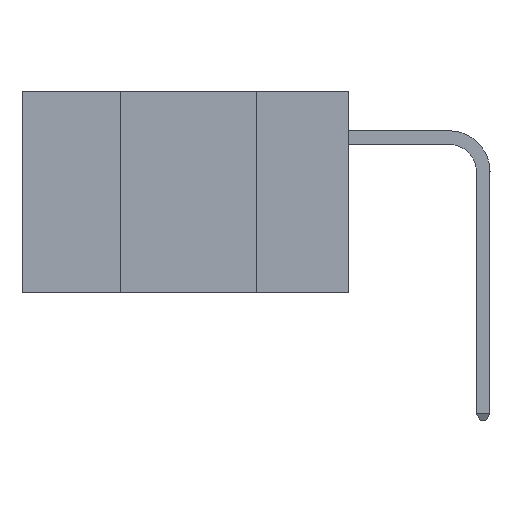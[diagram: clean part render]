
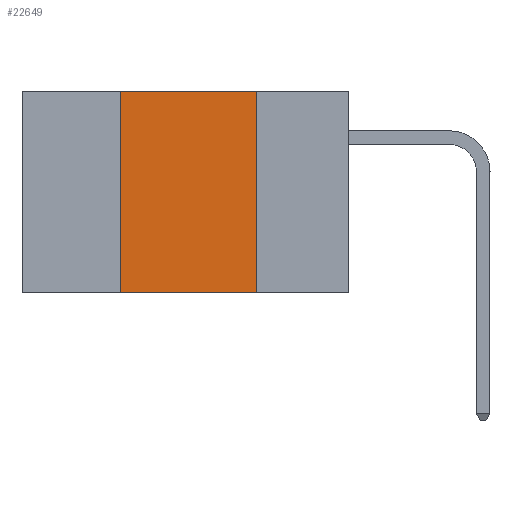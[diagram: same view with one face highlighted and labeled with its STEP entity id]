
A CAD part, left-side view. The second image highlights one B-rep face of the part: STEP entity #22649.
In plain terms, the highlighted planar face has unit normal (-1, 0, 0).
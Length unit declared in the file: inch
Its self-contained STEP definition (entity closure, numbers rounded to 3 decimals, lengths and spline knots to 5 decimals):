
#1308 = EDGE_CURVE ( 'NONE', #11373, #8260, #6706, .T. ) ;
#1594 = DIRECTION ( 'NONE',  ( 0., 0., -1. ) ) ;
#3029 = CARTESIAN_POINT ( 'NONE',  ( 0., 0.42, 0. ) ) ;
#3291 = VECTOR ( 'NONE', #25698, 39.37008 ) ;
#3367 = FACE_OUTER_BOUND ( 'NONE', #34215, .T. ) ;
#3496 = VERTEX_POINT ( 'NONE', #15528 ) ;
#5189 = ORIENTED_EDGE ( 'NONE', *, *, #33796, .F. ) ;
#6593 = DIRECTION ( 'NONE',  ( 0., -1., 0. ) ) ;
#6706 = LINE ( 'NONE', #19530, #32050 ) ;
#7103 = ORIENTED_EDGE ( 'NONE', *, *, #1308, .F. ) ;
#8260 = VERTEX_POINT ( 'NONE', #3029 ) ;
#8901 = AXIS2_PLACEMENT_3D ( 'NONE', #11120, #17249, #38572 ) ;
#11120 = CARTESIAN_POINT ( 'NONE',  ( 0., 0.6, 0. ) ) ;
#11373 = VERTEX_POINT ( 'NONE', #13842 ) ;
#13598 = CARTESIAN_POINT ( 'NONE',  ( 0., 0.6, -0.37 ) ) ;
#13842 = CARTESIAN_POINT ( 'NONE',  ( 0., 0.42, -0.37 ) ) ;
#13855 = LINE ( 'NONE', #34660, #20952 ) ;
#15528 = CARTESIAN_POINT ( 'NONE',  ( 0., 0.17, 0. ) ) ;
#17249 = DIRECTION ( 'NONE',  ( 1., 0., 0. ) ) ;
#19530 = CARTESIAN_POINT ( 'NONE',  ( 0., 0.42, 0. ) ) ;
#20952 = VECTOR ( 'NONE', #6593, 39.37008 ) ;
#22649 = ADVANCED_FACE ( 'NONE', ( #3367 ), #29400, .F. ) ;
#25698 = DIRECTION ( 'NONE',  ( 0., -1., 0. ) ) ;
#28758 = EDGE_CURVE ( 'NONE', #11373, #33150, #34875, .T. ) ;
#29241 = VECTOR ( 'NONE', #1594, 39.37008 ) ;
#29400 = PLANE ( 'NONE',  #8901 ) ;
#31492 = ORIENTED_EDGE ( 'NONE', *, *, #28758, .T. ) ;
#32050 = VECTOR ( 'NONE', #37795, 39.37008 ) ;
#32093 = EDGE_CURVE ( 'NONE', #3496, #33150, #37345, .T. ) ;
#33150 = VERTEX_POINT ( 'NONE', #34159 ) ;
#33796 = EDGE_CURVE ( 'NONE', #8260, #3496, #13855, .T. ) ;
#34159 = CARTESIAN_POINT ( 'NONE',  ( 0., 0.17, -0.37 ) ) ;
#34215 = EDGE_LOOP ( 'NONE', ( #36726, #5189, #7103, #31492 ) ) ;
#34660 = CARTESIAN_POINT ( 'NONE',  ( 0., 0.6, 0. ) ) ;
#34875 = LINE ( 'NONE', #13598, #3291 ) ;
#36726 = ORIENTED_EDGE ( 'NONE', *, *, #32093, .F. ) ;
#37345 = LINE ( 'NONE', #38228, #29241 ) ;
#37795 = DIRECTION ( 'NONE',  ( 0., 0., 1. ) ) ;
#38228 = CARTESIAN_POINT ( 'NONE',  ( 0., 0.17, 0. ) ) ;
#38572 = DIRECTION ( 'NONE',  ( 0., 0., -1. ) ) ;
